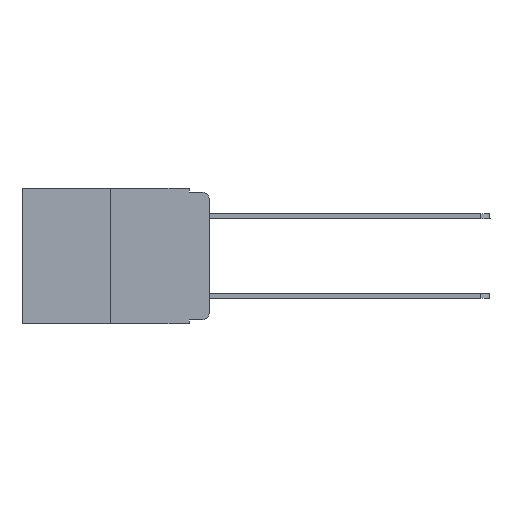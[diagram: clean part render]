
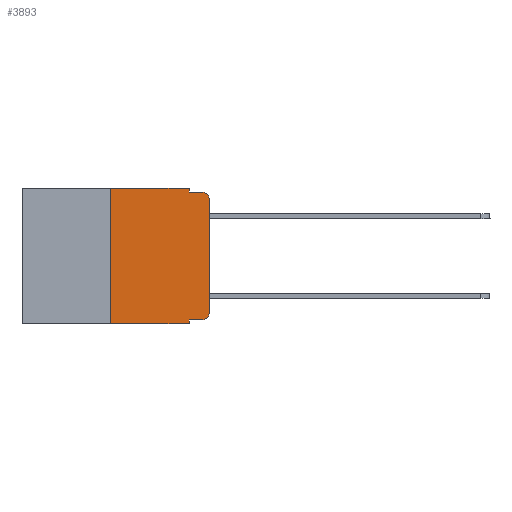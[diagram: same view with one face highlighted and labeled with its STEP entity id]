
A CAD part, left-side view. The second image highlights one B-rep face of the part: STEP entity #3893.
In plain terms, the highlighted planar face has unit normal (-1, 0, 0).
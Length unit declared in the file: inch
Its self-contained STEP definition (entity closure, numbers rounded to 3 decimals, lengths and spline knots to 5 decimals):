
#22 = CARTESIAN_POINT ( 'NONE',  ( 0., 0., -0.313 ) ) ;
#242 = CARTESIAN_POINT ( 'NONE',  ( 0., 0.473, 0. ) ) ;
#1030 = CARTESIAN_POINT ( 'NONE',  ( 0., 0.473, -0.343 ) ) ;
#1040 = CARTESIAN_POINT ( 'NONE',  ( 0., 0.25, -0.343 ) ) ;
#1127 = LINE ( 'NONE', #2577, #18604 ) ;
#1299 = ORIENTED_EDGE ( 'NONE', *, *, #18158, .F. ) ;
#1820 = EDGE_CURVE ( 'NONE', #20678, #21137, #14546, .T. ) ;
#1831 = CARTESIAN_POINT ( 'NONE',  ( 0., 0.02, -0.03 ) ) ;
#2430 = EDGE_CURVE ( 'NONE', #15967, #5403, #20311, .T. ) ;
#2458 = CARTESIAN_POINT ( 'NONE',  ( 0., 0.473, 0. ) ) ;
#2566 = PLANE ( 'NONE',  #18800 ) ;
#2577 = CARTESIAN_POINT ( 'NONE',  ( 0., 0.051, 0. ) ) ;
#2863 = CARTESIAN_POINT ( 'NONE',  ( 0., 0.051, -0.333 ) ) ;
#2878 = FACE_OUTER_BOUND ( 'NONE', #21639, .T. ) ;
#3383 = DIRECTION ( 'NONE',  ( 0., 0., 1. ) ) ;
#3893 = ADVANCED_FACE ( 'NONE', ( #2878 ), #2566, .F. ) ;
#4040 = VECTOR ( 'NONE', #7736, 39.37008 ) ;
#4086 = ORIENTED_EDGE ( 'NONE', *, *, #2430, .F. ) ;
#4309 = CARTESIAN_POINT ( 'NONE',  ( 0., 0., -0.03 ) ) ;
#4543 = CIRCLE ( 'NONE', #10130, 0.02 ) ;
#4604 = CARTESIAN_POINT ( 'NONE',  ( 0., 0.02, -0.333 ) ) ;
#5220 = CARTESIAN_POINT ( 'NONE',  ( 0., 0.051, 0. ) ) ;
#5374 = VERTEX_POINT ( 'NONE', #1040 ) ;
#5403 = VERTEX_POINT ( 'NONE', #8170 ) ;
#5505 = VERTEX_POINT ( 'NONE', #19973 ) ;
#6424 = ORIENTED_EDGE ( 'NONE', *, *, #21410, .F. ) ;
#6902 = DIRECTION ( 'NONE',  ( 0., 0., -1. ) ) ;
#7527 = LINE ( 'NONE', #15921, #10942 ) ;
#7711 = DIRECTION ( 'NONE',  ( 1., 0., 0. ) ) ;
#7736 = DIRECTION ( 'NONE',  ( 0., -1., 0. ) ) ;
#7764 = VECTOR ( 'NONE', #21233, 39.37008 ) ;
#8170 = CARTESIAN_POINT ( 'NONE',  ( 0., 0.051, -0.01 ) ) ;
#8320 = VECTOR ( 'NONE', #9790, 39.37008 ) ;
#8415 = LINE ( 'NONE', #9637, #16390 ) ;
#9468 = CARTESIAN_POINT ( 'NONE',  ( 0., 0.02, -0.313 ) ) ;
#9578 = DIRECTION ( 'NONE',  ( 0., 0., -1. ) ) ;
#9637 = CARTESIAN_POINT ( 'NONE',  ( 0., 0.25, 0. ) ) ;
#9790 = DIRECTION ( 'NONE',  ( 0., -1., 0. ) ) ;
#10130 = AXIS2_PLACEMENT_3D ( 'NONE', #1831, #15188, #6902 ) ;
#10535 = VERTEX_POINT ( 'NONE', #22 ) ;
#10892 = CIRCLE ( 'NONE', #14353, 0.02 ) ;
#10942 = VECTOR ( 'NONE', #18995, 39.37008 ) ;
#11047 = LINE ( 'NONE', #14526, #12224 ) ;
#12224 = VECTOR ( 'NONE', #17384, 39.37008 ) ;
#12325 = EDGE_CURVE ( 'NONE', #5374, #18977, #16038, .T. ) ;
#12516 = ORIENTED_EDGE ( 'NONE', *, *, #18400, .T. ) ;
#12785 = ORIENTED_EDGE ( 'NONE', *, *, #18456, .T. ) ;
#12957 = CARTESIAN_POINT ( 'NONE',  ( 0., 0.02, -0.01 ) ) ;
#12963 = DIRECTION ( 'NONE',  ( -1., 0., 0. ) ) ;
#13181 = CARTESIAN_POINT ( 'NONE',  ( 0., 0.051, 0. ) ) ;
#14077 = ORIENTED_EDGE ( 'NONE', *, *, #12325, .T. ) ;
#14084 = DIRECTION ( 'NONE',  ( 0., 0., -1. ) ) ;
#14269 = ORIENTED_EDGE ( 'NONE', *, *, #17336, .F. ) ;
#14280 = DIRECTION ( 'NONE',  ( 0., 0., -1. ) ) ;
#14353 = AXIS2_PLACEMENT_3D ( 'NONE', #9468, #12963, #9578 ) ;
#14526 = CARTESIAN_POINT ( 'NONE',  ( 0., 0., 0. ) ) ;
#14546 = LINE ( 'NONE', #19576, #7764 ) ;
#15158 = DIRECTION ( 'NONE',  ( 0., 0., -1. ) ) ;
#15188 = DIRECTION ( 'NONE',  ( -1., 0., 0. ) ) ;
#15487 = ORIENTED_EDGE ( 'NONE', *, *, #20171, .T. ) ;
#15824 = VERTEX_POINT ( 'NONE', #12957 ) ;
#15921 = CARTESIAN_POINT ( 'NONE',  ( 0., 0.051, -0.01 ) ) ;
#15967 = VERTEX_POINT ( 'NONE', #13181 ) ;
#16038 = LINE ( 'NONE', #1030, #4040 ) ;
#16309 = VERTEX_POINT ( 'NONE', #4309 ) ;
#16390 = VECTOR ( 'NONE', #3383, 39.37008 ) ;
#16613 = VECTOR ( 'NONE', #15158, 39.37008 ) ;
#16736 = ORIENTED_EDGE ( 'NONE', *, *, #21388, .F. ) ;
#17336 = EDGE_CURVE ( 'NONE', #5505, #15967, #20279, .T. ) ;
#17384 = DIRECTION ( 'NONE',  ( 0., 0., 1. ) ) ;
#17577 = CARTESIAN_POINT ( 'NONE',  ( 0., 0.051, -0.343 ) ) ;
#18158 = EDGE_CURVE ( 'NONE', #5374, #5505, #8415, .T. ) ;
#18400 = EDGE_CURVE ( 'NONE', #16309, #15824, #4543, .T. ) ;
#18456 = EDGE_CURVE ( 'NONE', #10535, #16309, #11047, .T. ) ;
#18604 = VECTOR ( 'NONE', #14084, 39.37008 ) ;
#18800 = AXIS2_PLACEMENT_3D ( 'NONE', #2458, #7711, #14280 ) ;
#18952 = ORIENTED_EDGE ( 'NONE', *, *, #1820, .T. ) ;
#18977 = VERTEX_POINT ( 'NONE', #17577 ) ;
#18995 = DIRECTION ( 'NONE',  ( 0., -1., 0. ) ) ;
#19576 = CARTESIAN_POINT ( 'NONE',  ( 0., 0.051, -0.333 ) ) ;
#19973 = CARTESIAN_POINT ( 'NONE',  ( 0., 0.25, 0. ) ) ;
#20171 = EDGE_CURVE ( 'NONE', #21137, #10535, #10892, .T. ) ;
#20279 = LINE ( 'NONE', #242, #8320 ) ;
#20311 = LINE ( 'NONE', #5220, #16613 ) ;
#20678 = VERTEX_POINT ( 'NONE', #2863 ) ;
#21137 = VERTEX_POINT ( 'NONE', #4604 ) ;
#21233 = DIRECTION ( 'NONE',  ( 0., -1., 0. ) ) ;
#21388 = EDGE_CURVE ( 'NONE', #20678, #18977, #1127, .T. ) ;
#21410 = EDGE_CURVE ( 'NONE', #5403, #15824, #7527, .T. ) ;
#21639 = EDGE_LOOP ( 'NONE', ( #12785, #12516, #6424, #4086, #14269, #1299, #14077, #16736, #18952, #15487 ) ) ;
